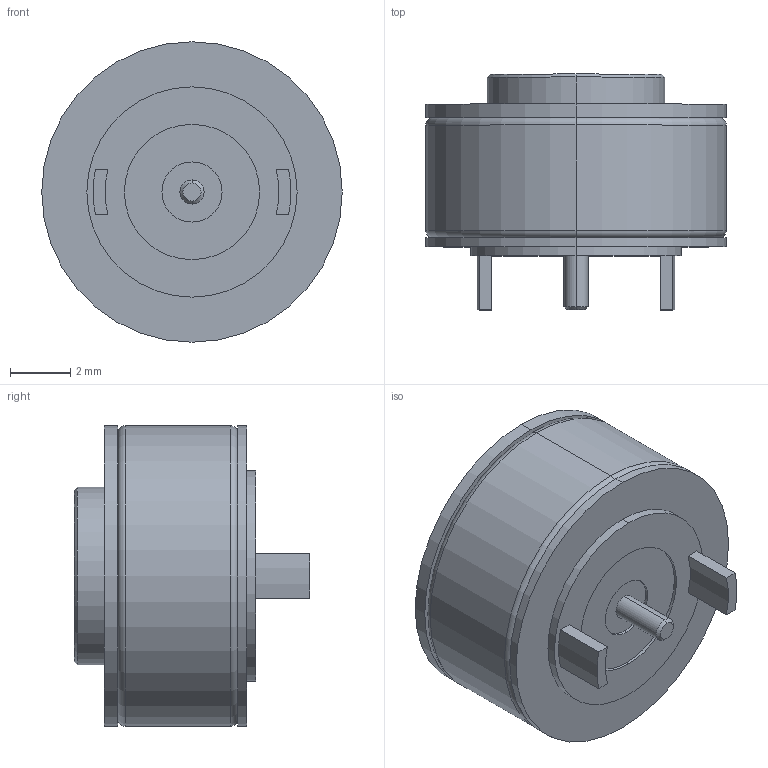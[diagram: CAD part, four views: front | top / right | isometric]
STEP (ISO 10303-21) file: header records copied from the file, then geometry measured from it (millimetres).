
FILE_DESCRIPTION (( 'STEP AP203' ), '1' );
FILE_NAME ('686-B03222011D1-NEW.STEP', '2023-02-10T12:14:34', ( '' ), ( '' ), 'SwSTEP 2.0', 'SolidWorks 2020', '' );
FILE_SCHEMA (( 'CONFIG_CONTROL_DESIGN' ));
Length unit declared in the file: millimetre
Products named in the file (1): 686-B03222011D1-NEW
Bounding box: 10 x 7.85 x 10 mm (x, y, z)
Volume: 411.7 mm3; surface area: 375.9 mm2
Topology: 1 solids, 1 shells, 49 faces, 100 edges, 64 vertices
Faces by surface type: cylinder 22, plane 17, cone 6, torus 4
Entity records: 1387 total; most frequent: DIRECTION 260, CARTESIAN_POINT 214, ORIENTED_EDGE 200, AXIS2_PLACEMENT_3D 110, EDGE_CURVE 100, VERTEX_POINT 64, EDGE_LOOP 60, CIRCLE 60
